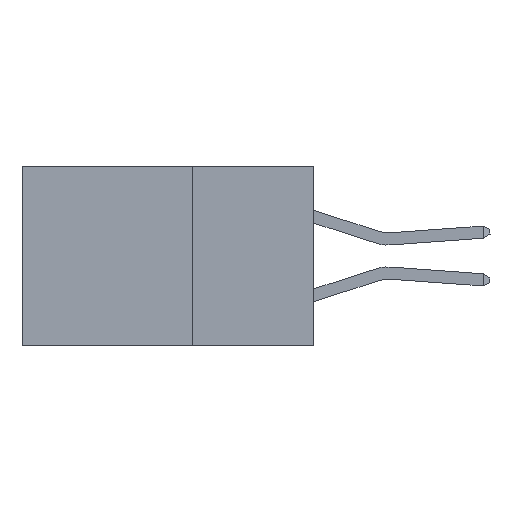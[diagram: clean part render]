
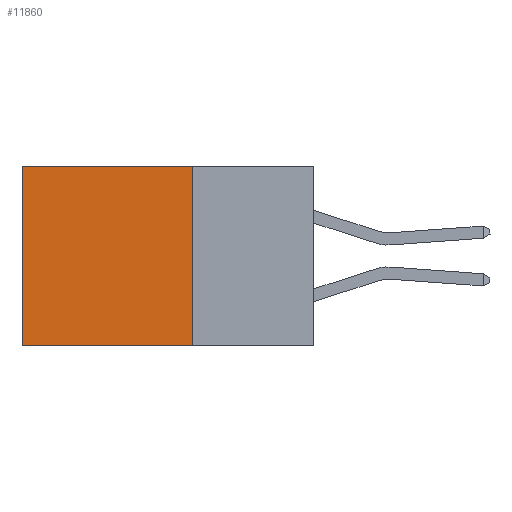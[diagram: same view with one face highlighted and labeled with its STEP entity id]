
A CAD part, left-side view. The second image highlights one B-rep face of the part: STEP entity #11860.
In plain terms, the highlighted planar face has unit normal (-1, 0, 0).
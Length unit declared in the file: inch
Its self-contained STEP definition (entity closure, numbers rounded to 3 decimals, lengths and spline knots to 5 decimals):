
#192 = VECTOR ( 'NONE', #7632, 39.37008 ) ;
#422 = DIRECTION ( 'NONE',  ( 0., 0., -1. ) ) ;
#779 = FACE_OUTER_BOUND ( 'NONE', #10388, .T. ) ;
#941 = LINE ( 'NONE', #19300, #192 ) ;
#1370 = VECTOR ( 'NONE', #422, 39.37008 ) ;
#1995 = VECTOR ( 'NONE', #23838, 39.37008 ) ;
#3295 = ORIENTED_EDGE ( 'NONE', *, *, #27030, .T. ) ;
#3793 = ORIENTED_EDGE ( 'NONE', *, *, #20198, .T. ) ;
#4265 = ORIENTED_EDGE ( 'NONE', *, *, #27150, .F. ) ;
#7494 = AXIS2_PLACEMENT_3D ( 'NONE', #18042, #22705, #8725 ) ;
#7632 = DIRECTION ( 'NONE',  ( 0., 0., -1. ) ) ;
#8548 = CARTESIAN_POINT ( 'NONE',  ( 0.2875, 0.25, 0. ) ) ;
#8725 = DIRECTION ( 'NONE',  ( 0., 0., -1. ) ) ;
#9087 = LINE ( 'NONE', #9785, #1995 ) ;
#9785 = CARTESIAN_POINT ( 'NONE',  ( 0.2875, 0.25, 0. ) ) ;
#10307 = VECTOR ( 'NONE', #28906, 39.37008 ) ;
#10388 = EDGE_LOOP ( 'NONE', ( #3295, #4265, #22035, #3793 ) ) ;
#10642 = VERTEX_POINT ( 'NONE', #25170 ) ;
#11231 = VERTEX_POINT ( 'NONE', #8548 ) ;
#11860 = ADVANCED_FACE ( 'NONE', ( #779 ), #27244, .F. ) ;
#12289 = CARTESIAN_POINT ( 'NONE',  ( 0.2875, 0.6, 0. ) ) ;
#12310 = VERTEX_POINT ( 'NONE', #26501 ) ;
#16855 = CARTESIAN_POINT ( 'NONE',  ( 0.2875, 0.6, -0.37 ) ) ;
#18042 = CARTESIAN_POINT ( 'NONE',  ( 0.2875, 0.25, 0. ) ) ;
#19300 = CARTESIAN_POINT ( 'NONE',  ( 0.2875, 0.25, 0. ) ) ;
#20185 = LINE ( 'NONE', #12289, #1370 ) ;
#20198 = EDGE_CURVE ( 'NONE', #11231, #10642, #9087, .T. ) ;
#22035 = ORIENTED_EDGE ( 'NONE', *, *, #27723, .F. ) ;
#22705 = DIRECTION ( 'NONE',  ( 1., 0., 0. ) ) ;
#23838 = DIRECTION ( 'NONE',  ( 0., 1., 0. ) ) ;
#25170 = CARTESIAN_POINT ( 'NONE',  ( 0.2875, 0.6, 0. ) ) ;
#25794 = VERTEX_POINT ( 'NONE', #16855 ) ;
#26501 = CARTESIAN_POINT ( 'NONE',  ( 0.2875, 0.25, -0.37 ) ) ;
#26583 = CARTESIAN_POINT ( 'NONE',  ( 0.2875, 0.25, -0.37 ) ) ;
#27030 = EDGE_CURVE ( 'NONE', #10642, #25794, #20185, .T. ) ;
#27150 = EDGE_CURVE ( 'NONE', #12310, #25794, #28839, .T. ) ;
#27244 = PLANE ( 'NONE',  #7494 ) ;
#27723 = EDGE_CURVE ( 'NONE', #11231, #12310, #941, .T. ) ;
#28839 = LINE ( 'NONE', #26583, #10307 ) ;
#28906 = DIRECTION ( 'NONE',  ( 0., 1., 0. ) ) ;
